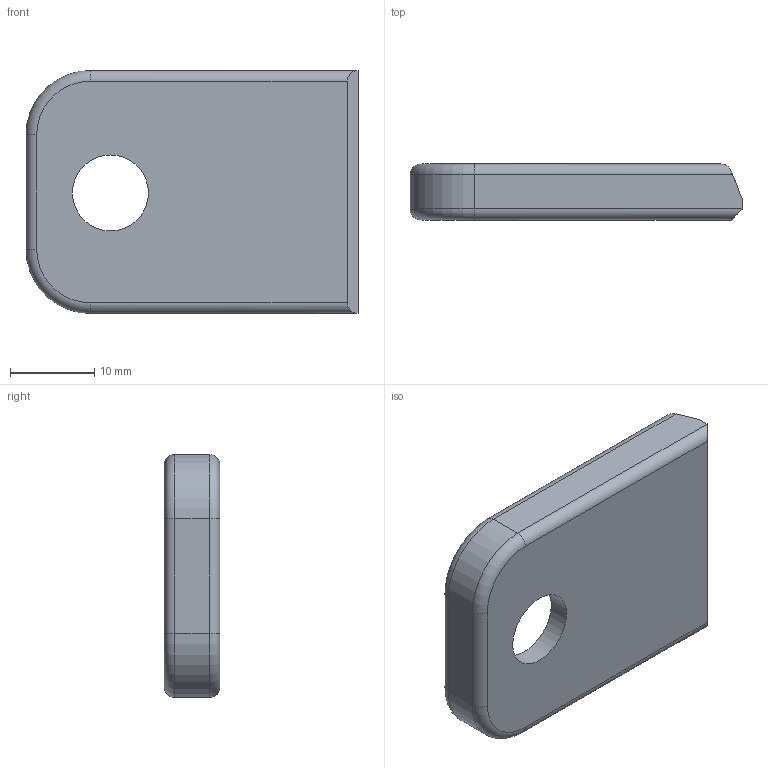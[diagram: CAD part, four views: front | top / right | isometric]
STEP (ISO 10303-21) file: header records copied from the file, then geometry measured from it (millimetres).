
FILE_DESCRIPTION(('FreeCAD Model'),'2;1');
FILE_NAME('baseplate.step', '2019-10-17T20:30:17',('Author'),(''), 'Open CASCADE STEP processor 7.3','FreeCAD','Unknown');
FILE_SCHEMA(('AUTOMOTIVE_DESIGN { 1 0 10303 214 1 1 1 1 }'));
Length unit declared in the file: millimetre
Products named in the file (1): Cut
Bounding box: 39.32 x 6.6 x 28.78 mm (x, y, z)
Volume: 3434.7 mm3; surface area: 3406.5 mm2
Topology: 1 solids, 1 shells, 64 faces, 154 edges, 92 vertices
Faces by surface type: cylinder 31, plane 19, torus 10, bspline 4
Full cylindrical faces by diameter (mm): 9 x1
Entity records: 5163 total; most frequent: CARTESIAN_POINT 1664, DIRECTION 567, ORIENTED_EDGE 308, PCURVE 308, DEFINITIONAL_REPRESENTATION 308, LINE 304, VECTOR 304, EDGE_CURVE 154
